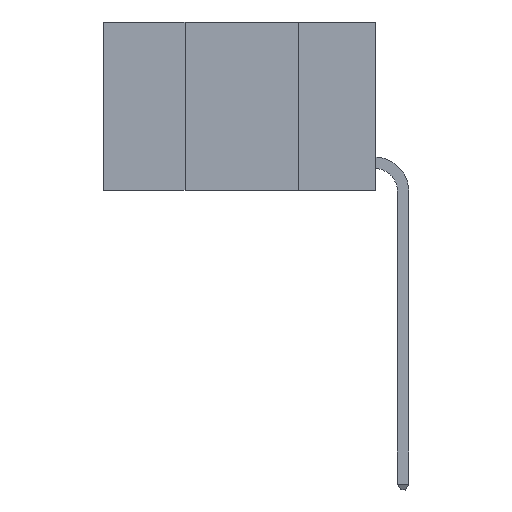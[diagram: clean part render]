
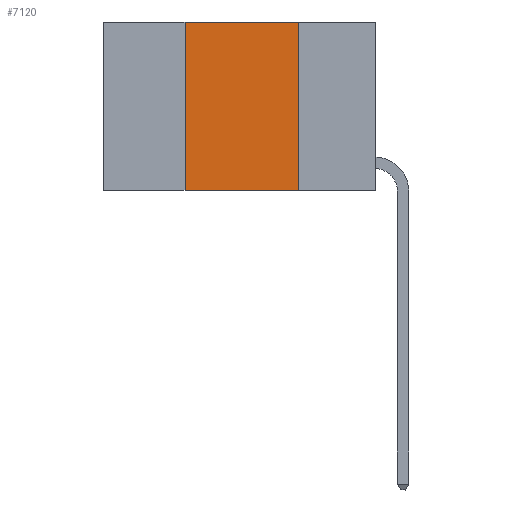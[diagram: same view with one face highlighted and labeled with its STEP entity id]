
A CAD part, left-side view. The second image highlights one B-rep face of the part: STEP entity #7120.
In plain terms, the highlighted planar face has unit normal (-1, 0, 0).
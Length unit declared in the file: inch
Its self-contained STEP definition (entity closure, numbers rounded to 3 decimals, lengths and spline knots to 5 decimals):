
#15 = CARTESIAN_POINT ( 'NONE',  ( 0., 0.42, 0. ) ) ;
#198 = ORIENTED_EDGE ( 'NONE', *, *, #16280, .F. ) ;
#554 = EDGE_CURVE ( 'NONE', #22954, #15111, #2540, .T. ) ;
#805 = ORIENTED_EDGE ( 'NONE', *, *, #5643, .T. ) ;
#1831 = EDGE_CURVE ( 'NONE', #10982, #1987, #4870, .T. ) ;
#1987 = VERTEX_POINT ( 'NONE', #17242 ) ;
#2082 = CARTESIAN_POINT ( 'NONE',  ( 0., 0.6, 0. ) ) ;
#2428 = LINE ( 'NONE', #15568, #7463 ) ;
#2540 = LINE ( 'NONE', #18412, #7575 ) ;
#3234 = CARTESIAN_POINT ( 'NONE',  ( 0., 0.42, -0.37 ) ) ;
#3634 = DIRECTION ( 'NONE',  ( 0., 0., -1. ) ) ;
#4870 = LINE ( 'NONE', #15, #9224 ) ;
#5062 = FACE_OUTER_BOUND ( 'NONE', #14499, .T. ) ;
#5586 = DIRECTION ( 'NONE',  ( 0., 0., 1. ) ) ;
#5643 = EDGE_CURVE ( 'NONE', #10982, #15111, #2428, .T. ) ;
#7120 = ADVANCED_FACE ( 'NONE', ( #5062 ), #23695, .F. ) ;
#7463 = VECTOR ( 'NONE', #10022, 39.37008 ) ;
#7575 = VECTOR ( 'NONE', #17270, 39.37008 ) ;
#9224 = VECTOR ( 'NONE', #5586, 39.37008 ) ;
#10022 = DIRECTION ( 'NONE',  ( 0., -1., 0. ) ) ;
#10982 = VERTEX_POINT ( 'NONE', #3234 ) ;
#11574 = LINE ( 'NONE', #2082, #12167 ) ;
#12167 = VECTOR ( 'NONE', #15076, 39.37008 ) ;
#12288 = AXIS2_PLACEMENT_3D ( 'NONE', #12863, #14719, #3634 ) ;
#12863 = CARTESIAN_POINT ( 'NONE',  ( 0., 0.6, 0. ) ) ;
#14499 = EDGE_LOOP ( 'NONE', ( #14525, #198, #15086, #805 ) ) ;
#14525 = ORIENTED_EDGE ( 'NONE', *, *, #554, .F. ) ;
#14719 = DIRECTION ( 'NONE',  ( 1., 0., 0. ) ) ;
#15076 = DIRECTION ( 'NONE',  ( 0., -1., 0. ) ) ;
#15086 = ORIENTED_EDGE ( 'NONE', *, *, #1831, .F. ) ;
#15111 = VERTEX_POINT ( 'NONE', #22852 ) ;
#15568 = CARTESIAN_POINT ( 'NONE',  ( 0., 0.6, -0.37 ) ) ;
#16280 = EDGE_CURVE ( 'NONE', #1987, #22954, #11574, .T. ) ;
#16439 = CARTESIAN_POINT ( 'NONE',  ( 0., 0.17, 0. ) ) ;
#17242 = CARTESIAN_POINT ( 'NONE',  ( 0., 0.42, 0. ) ) ;
#17270 = DIRECTION ( 'NONE',  ( 0., 0., -1. ) ) ;
#18412 = CARTESIAN_POINT ( 'NONE',  ( 0., 0.17, 0. ) ) ;
#22852 = CARTESIAN_POINT ( 'NONE',  ( 0., 0.17, -0.37 ) ) ;
#22954 = VERTEX_POINT ( 'NONE', #16439 ) ;
#23695 = PLANE ( 'NONE',  #12288 ) ;
